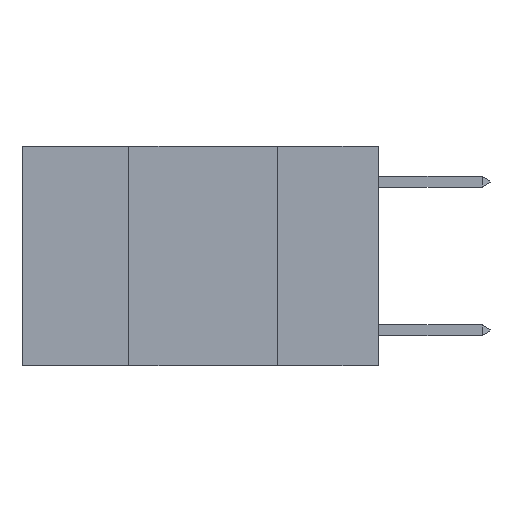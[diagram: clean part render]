
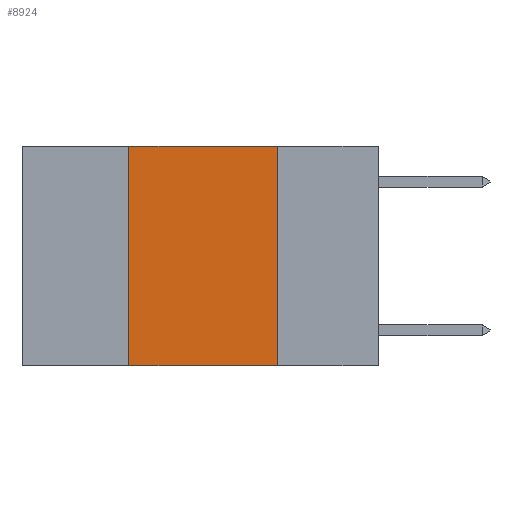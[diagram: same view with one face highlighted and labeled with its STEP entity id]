
A CAD part, left-side view. The second image highlights one B-rep face of the part: STEP entity #8924.
In plain terms, the highlighted planar face has unit normal (-1, 0, 0).
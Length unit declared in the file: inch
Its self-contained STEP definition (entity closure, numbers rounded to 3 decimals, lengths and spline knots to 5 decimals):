
#193 = VECTOR ( 'NONE', #4860, 39.37008 ) ;
#541 = LINE ( 'NONE', #6481, #17607 ) ;
#834 = DIRECTION ( 'NONE',  ( 0., 0., -1. ) ) ;
#2953 = EDGE_CURVE ( 'NONE', #12604, #17313, #541, .T. ) ;
#3521 = EDGE_CURVE ( 'NONE', #22139, #12604, #23204, .T. ) ;
#3770 = ORIENTED_EDGE ( 'NONE', *, *, #3521, .F. ) ;
#4234 = CARTESIAN_POINT ( 'NONE',  ( 0., 0.42, 0. ) ) ;
#4845 = CARTESIAN_POINT ( 'NONE',  ( 0., 0.42, -0.37 ) ) ;
#4860 = DIRECTION ( 'NONE',  ( 0., -1., 0. ) ) ;
#5269 = EDGE_CURVE ( 'NONE', #14082, #22139, #22859, .T. ) ;
#6481 = CARTESIAN_POINT ( 'NONE',  ( 0., 0.17, 0. ) ) ;
#7400 = CARTESIAN_POINT ( 'NONE',  ( 0., 0.17, 0. ) ) ;
#7870 = CARTESIAN_POINT ( 'NONE',  ( 0., 0.6, -0.37 ) ) ;
#8924 = ADVANCED_FACE ( 'NONE', ( #17452 ), #20995, .F. ) ;
#11238 = EDGE_CURVE ( 'NONE', #14082, #17313, #15279, .T. ) ;
#11748 = DIRECTION ( 'NONE',  ( 0., -1., 0. ) ) ;
#11986 = DIRECTION ( 'NONE',  ( 1., 0., 0. ) ) ;
#12155 = CARTESIAN_POINT ( 'NONE',  ( 0., 0.42, 0. ) ) ;
#12361 = CARTESIAN_POINT ( 'NONE',  ( 0., 0.17, -0.37 ) ) ;
#12604 = VERTEX_POINT ( 'NONE', #7400 ) ;
#13292 = ORIENTED_EDGE ( 'NONE', *, *, #2953, .F. ) ;
#13849 = DIRECTION ( 'NONE',  ( 0., 0., 1. ) ) ;
#14035 = CARTESIAN_POINT ( 'NONE',  ( 0., 0.6, 0. ) ) ;
#14082 = VERTEX_POINT ( 'NONE', #4845 ) ;
#14642 = ORIENTED_EDGE ( 'NONE', *, *, #5269, .F. ) ;
#15279 = LINE ( 'NONE', #7870, #20836 ) ;
#15885 = ORIENTED_EDGE ( 'NONE', *, *, #11238, .T. ) ;
#17313 = VERTEX_POINT ( 'NONE', #12361 ) ;
#17452 = FACE_OUTER_BOUND ( 'NONE', #18599, .T. ) ;
#17607 = VECTOR ( 'NONE', #19342, 39.37008 ) ;
#17829 = CARTESIAN_POINT ( 'NONE',  ( 0., 0.6, 0. ) ) ;
#18599 = EDGE_LOOP ( 'NONE', ( #13292, #3770, #14642, #15885 ) ) ;
#19342 = DIRECTION ( 'NONE',  ( 0., 0., -1. ) ) ;
#19964 = AXIS2_PLACEMENT_3D ( 'NONE', #14035, #11986, #834 ) ;
#20836 = VECTOR ( 'NONE', #11748, 39.37008 ) ;
#20995 = PLANE ( 'NONE',  #19964 ) ;
#21322 = VECTOR ( 'NONE', #13849, 39.37008 ) ;
#22139 = VERTEX_POINT ( 'NONE', #4234 ) ;
#22859 = LINE ( 'NONE', #12155, #21322 ) ;
#23204 = LINE ( 'NONE', #17829, #193 ) ;
